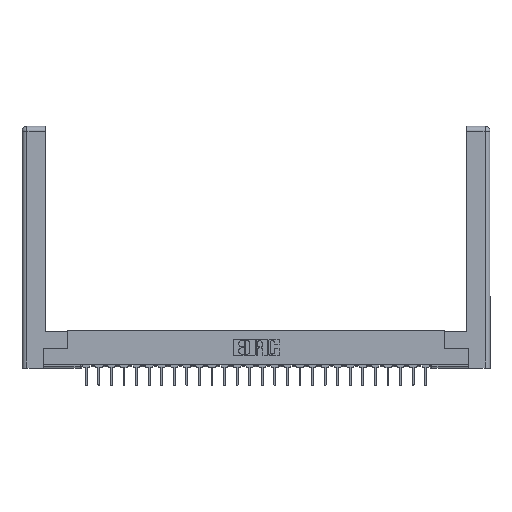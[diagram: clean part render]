
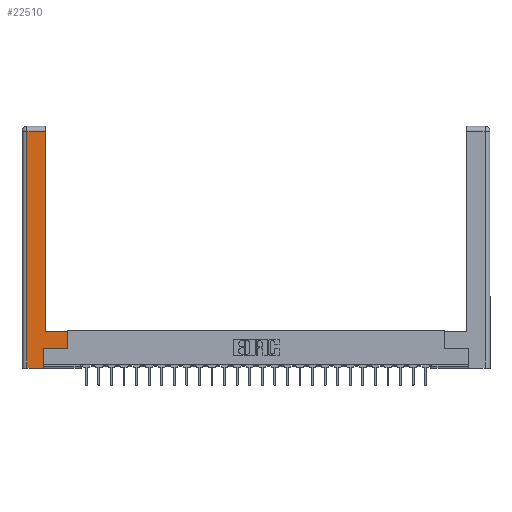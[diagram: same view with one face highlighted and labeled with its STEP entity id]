
A CAD part, top view. The second image highlights one B-rep face of the part: STEP entity #22510.
In plain terms, the highlighted planar face has unit normal (0, 0, 1).
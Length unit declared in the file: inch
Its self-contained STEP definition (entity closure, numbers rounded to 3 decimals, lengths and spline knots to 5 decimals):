
#844 = DIRECTION ( 'NONE',  ( -1., 0., 0. ) ) ;
#1258 = DIRECTION ( 'NONE',  ( 1., 0., 0. ) ) ;
#1291 = CARTESIAN_POINT ( 'NONE',  ( 0.265, 0.245, 0. ) ) ;
#1330 = ORIENTED_EDGE ( 'NONE', *, *, #19345, .T. ) ;
#1413 = CARTESIAN_POINT ( 'NONE',  ( 0.295, 0.45, 0. ) ) ;
#2152 = LINE ( 'NONE', #14781, #17608 ) ;
#2592 = EDGE_CURVE ( 'NONE', #25548, #10721, #27357, .T. ) ;
#3538 = ORIENTED_EDGE ( 'NONE', *, *, #26325, .T. ) ;
#3727 = EDGE_CURVE ( 'NONE', #22923, #9440, #13473, .T. ) ;
#4724 = VECTOR ( 'NONE', #844, 39.37008 ) ;
#5159 = CARTESIAN_POINT ( 'NONE',  ( 0.265, 0., 0. ) ) ;
#5705 = CARTESIAN_POINT ( 'NONE',  ( 0.565, 0.245, 0. ) ) ;
#5773 = CARTESIAN_POINT ( 'NONE',  ( 0.565, 0.45, 0. ) ) ;
#5820 = EDGE_CURVE ( 'NONE', #26587, #8870, #10005, .T. ) ;
#6339 = DIRECTION ( 'NONE',  ( 0., 1., 0. ) ) ;
#6698 = PLANE ( 'NONE',  #17005 ) ;
#6758 = CARTESIAN_POINT ( 'NONE',  ( 0.0615, 2.94, 0. ) ) ;
#7811 = VERTEX_POINT ( 'NONE', #24446 ) ;
#8631 = CARTESIAN_POINT ( 'NONE',  ( 0.295, 3., 0. ) ) ;
#8870 = VERTEX_POINT ( 'NONE', #6758 ) ;
#9440 = VERTEX_POINT ( 'NONE', #20591 ) ;
#9850 = ORIENTED_EDGE ( 'NONE', *, *, #2592, .T. ) ;
#10005 = LINE ( 'NONE', #14328, #4724 ) ;
#10354 = VERTEX_POINT ( 'NONE', #27514 ) ;
#10577 = EDGE_LOOP ( 'NONE', ( #1330, #15532, #3538, #17243, #28031, #9850, #18056, #21478 ) ) ;
#10707 = FACE_OUTER_BOUND ( 'NONE', #10577, .T. ) ;
#10721 = VERTEX_POINT ( 'NONE', #13745 ) ;
#11601 = CARTESIAN_POINT ( 'NONE',  ( 0.295, 2.94, 0. ) ) ;
#11952 = LINE ( 'NONE', #5773, #25730 ) ;
#12332 = LINE ( 'NONE', #1291, #13445 ) ;
#12646 = LINE ( 'NONE', #8631, #20824 ) ;
#13445 = VECTOR ( 'NONE', #25095, 39.37008 ) ;
#13473 = LINE ( 'NONE', #5159, #14222 ) ;
#13745 = CARTESIAN_POINT ( 'NONE',  ( 0.565, 0.245, 0. ) ) ;
#14222 = VECTOR ( 'NONE', #17946, 39.37008 ) ;
#14328 = CARTESIAN_POINT ( 'NONE',  ( 0.0615, 2.94, 0. ) ) ;
#14781 = CARTESIAN_POINT ( 'NONE',  ( 0.0615, 0., 0. ) ) ;
#14964 = EDGE_CURVE ( 'NONE', #10721, #10354, #11952, .T. ) ;
#15327 = DIRECTION ( 'NONE',  ( -1., 0., 0. ) ) ;
#15532 = ORIENTED_EDGE ( 'NONE', *, *, #5820, .T. ) ;
#16210 = VECTOR ( 'NONE', #23358, 39.37008 ) ;
#17005 = AXIS2_PLACEMENT_3D ( 'NONE', #23748, #19471, #15327 ) ;
#17088 = EDGE_CURVE ( 'NONE', #10354, #7811, #25636, .T. ) ;
#17243 = ORIENTED_EDGE ( 'NONE', *, *, #3727, .T. ) ;
#17608 = VECTOR ( 'NONE', #23516, 39.37008 ) ;
#17733 = CARTESIAN_POINT ( 'NONE',  ( 0.265, 0.245, 0. ) ) ;
#17946 = DIRECTION ( 'NONE',  ( 1., 0., 0. ) ) ;
#18056 = ORIENTED_EDGE ( 'NONE', *, *, #14964, .T. ) ;
#19345 = EDGE_CURVE ( 'NONE', #7811, #26587, #12646, .T. ) ;
#19471 = DIRECTION ( 'NONE',  ( 0., 0., -1. ) ) ;
#19747 = VECTOR ( 'NONE', #1258, 39.37008 ) ;
#20591 = CARTESIAN_POINT ( 'NONE',  ( 0.265, 0., 0. ) ) ;
#20824 = VECTOR ( 'NONE', #6339, 39.37008 ) ;
#21478 = ORIENTED_EDGE ( 'NONE', *, *, #17088, .T. ) ;
#22510 = ADVANCED_FACE ( 'NONE', ( #10707 ), #6698, .F. ) ;
#22568 = DIRECTION ( 'NONE',  ( 0., 1., 0. ) ) ;
#22923 = VERTEX_POINT ( 'NONE', #26961 ) ;
#23358 = DIRECTION ( 'NONE',  ( -1., 0., 0. ) ) ;
#23516 = DIRECTION ( 'NONE',  ( 0., -1., 0. ) ) ;
#23748 = CARTESIAN_POINT ( 'NONE',  ( 0., 0., 0. ) ) ;
#24446 = CARTESIAN_POINT ( 'NONE',  ( 0.295, 0.45, 0. ) ) ;
#25095 = DIRECTION ( 'NONE',  ( 0., 1., 0. ) ) ;
#25548 = VERTEX_POINT ( 'NONE', #17733 ) ;
#25636 = LINE ( 'NONE', #1413, #16210 ) ;
#25730 = VECTOR ( 'NONE', #22568, 39.37008 ) ;
#26214 = EDGE_CURVE ( 'NONE', #9440, #25548, #12332, .T. ) ;
#26325 = EDGE_CURVE ( 'NONE', #8870, #22923, #2152, .T. ) ;
#26587 = VERTEX_POINT ( 'NONE', #11601 ) ;
#26961 = CARTESIAN_POINT ( 'NONE',  ( 0.0615, 0., 0. ) ) ;
#27357 = LINE ( 'NONE', #5705, #19747 ) ;
#27514 = CARTESIAN_POINT ( 'NONE',  ( 0.565, 0.45, 0. ) ) ;
#28031 = ORIENTED_EDGE ( 'NONE', *, *, #26214, .T. ) ;
